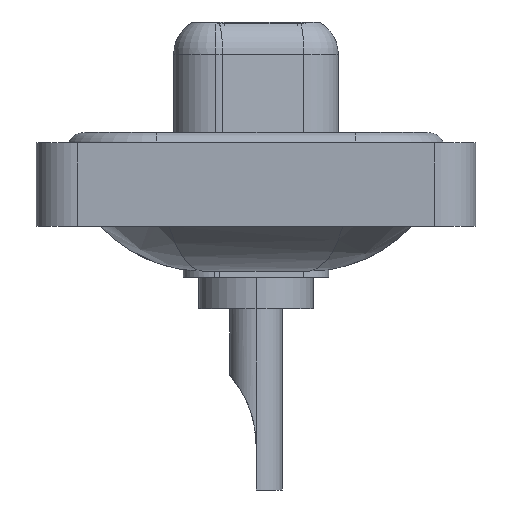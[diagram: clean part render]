
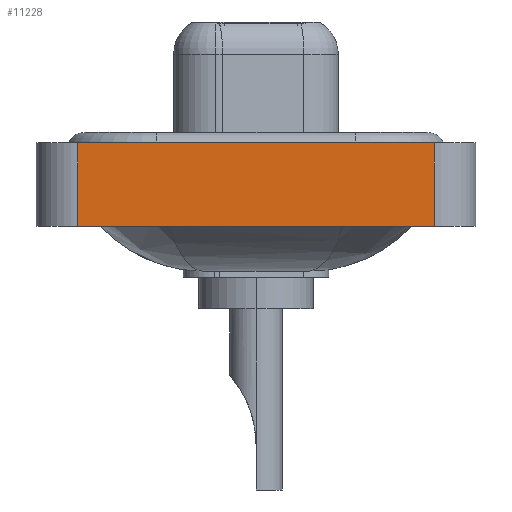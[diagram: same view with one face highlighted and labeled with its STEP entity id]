
A CAD part, left-side view. The second image highlights one B-rep face of the part: STEP entity #11228.
In plain terms, the highlighted planar face has unit normal (-1, 0, 0).
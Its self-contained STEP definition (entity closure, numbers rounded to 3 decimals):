
#914 = DIRECTION ( 'NONE',  ( 0., -1., 0. ) ) ;
#1166 = ORIENTED_EDGE ( 'NONE', *, *, #1441, .F. ) ;
#1441 = EDGE_CURVE ( 'NONE', #12565, #4615, #15796, .T. ) ;
#3286 = LINE ( 'NONE', #8688, #11770 ) ;
#3399 = DIRECTION ( 'NONE',  ( 0., -1., 0. ) ) ;
#3614 = CARTESIAN_POINT ( 'NONE',  ( -7.25, 8.55, 0.4 ) ) ;
#4615 = VERTEX_POINT ( 'NONE', #3614 ) ;
#4720 = LINE ( 'NONE', #10056, #5713 ) ;
#5259 = FACE_OUTER_BOUND ( 'NONE', #6973, .T. ) ;
#5713 = VECTOR ( 'NONE', #3399, 1000. ) ;
#6973 = EDGE_LOOP ( 'NONE', ( #16885, #9791, #1166, #12119 ) ) ;
#7123 = EDGE_CURVE ( 'NONE', #4615, #10414, #4720, .T. ) ;
#8595 = VERTEX_POINT ( 'NONE', #11628 ) ;
#8688 = CARTESIAN_POINT ( 'NONE',  ( -7.25, -8.55, -3.6 ) ) ;
#9205 = DIRECTION ( 'NONE',  ( 0., 0., 1. ) ) ;
#9535 = DIRECTION ( 'NONE',  ( -1., 0., 0. ) ) ;
#9755 = CARTESIAN_POINT ( 'NONE',  ( -7.25, -8.55, 0.4 ) ) ;
#9791 = ORIENTED_EDGE ( 'NONE', *, *, #7123, .F. ) ;
#10056 = CARTESIAN_POINT ( 'NONE',  ( -7.25, -8.55, 0.4 ) ) ;
#10197 = CARTESIAN_POINT ( 'NONE',  ( -7.25, -8.55, -3.6 ) ) ;
#10414 = VERTEX_POINT ( 'NONE', #9755 ) ;
#10876 = CARTESIAN_POINT ( 'NONE',  ( -7.25, -8.55, -3.6 ) ) ;
#11228 = ADVANCED_FACE ( 'NONE', ( #5259 ), #13433, .T. ) ;
#11628 = CARTESIAN_POINT ( 'NONE',  ( -7.25, -8.55, -3.6 ) ) ;
#11770 = VECTOR ( 'NONE', #16610, 1000. ) ;
#11843 = CARTESIAN_POINT ( 'NONE',  ( -7.25, 8.55, -3.6 ) ) ;
#12119 = ORIENTED_EDGE ( 'NONE', *, *, #12276, .T. ) ;
#12276 = EDGE_CURVE ( 'NONE', #12565, #8595, #17220, .T. ) ;
#12313 = AXIS2_PLACEMENT_3D ( 'NONE', #10876, #9535, #14911 ) ;
#12565 = VERTEX_POINT ( 'NONE', #12714 ) ;
#12714 = CARTESIAN_POINT ( 'NONE',  ( -7.25, 8.55, -3.6 ) ) ;
#13389 = EDGE_CURVE ( 'NONE', #8595, #10414, #3286, .T. ) ;
#13433 = PLANE ( 'NONE',  #12313 ) ;
#14911 = DIRECTION ( 'NONE',  ( 0., 0., 1. ) ) ;
#15796 = LINE ( 'NONE', #11843, #16395 ) ;
#16239 = VECTOR ( 'NONE', #914, 1000. ) ;
#16395 = VECTOR ( 'NONE', #9205, 1000. ) ;
#16610 = DIRECTION ( 'NONE',  ( 0., 0., 1. ) ) ;
#16885 = ORIENTED_EDGE ( 'NONE', *, *, #13389, .T. ) ;
#17220 = LINE ( 'NONE', #10197, #16239 ) ;
